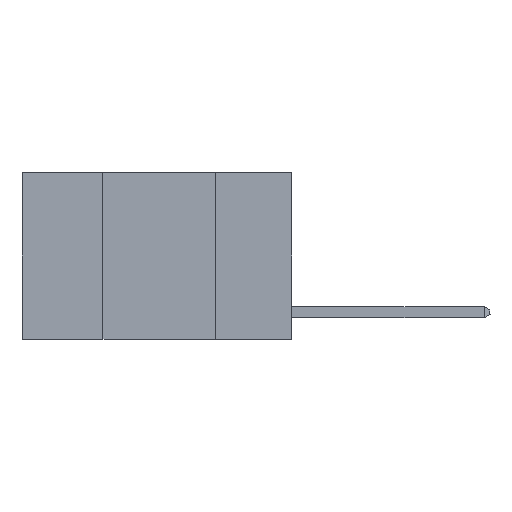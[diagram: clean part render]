
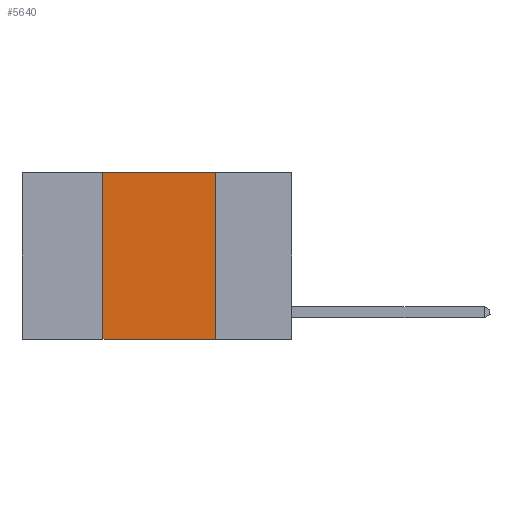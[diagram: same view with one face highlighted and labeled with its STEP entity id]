
A CAD part, left-side view. The second image highlights one B-rep face of the part: STEP entity #5640.
In plain terms, the highlighted planar face has unit normal (-1, 0, 0).
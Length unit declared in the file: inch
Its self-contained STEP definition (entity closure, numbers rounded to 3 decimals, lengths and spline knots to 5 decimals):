
#360 = EDGE_CURVE ( 'NONE', #12154, #3859, #1689, .T. ) ;
#563 = PLANE ( 'NONE',  #15640 ) ;
#622 = CARTESIAN_POINT ( 'NONE',  ( 0., 0.6, 0. ) ) ;
#1076 = DIRECTION ( 'NONE',  ( 0., 0., -1. ) ) ;
#1689 = LINE ( 'NONE', #13820, #8834 ) ;
#1871 = ORIENTED_EDGE ( 'NONE', *, *, #8017, .F. ) ;
#1886 = FACE_OUTER_BOUND ( 'NONE', #17137, .T. ) ;
#2322 = ORIENTED_EDGE ( 'NONE', *, *, #3202, .F. ) ;
#3202 = EDGE_CURVE ( 'NONE', #12154, #18218, #9195, .T. ) ;
#3463 = DIRECTION ( 'NONE',  ( 0., 0., -1. ) ) ;
#3859 = VERTEX_POINT ( 'NONE', #6863 ) ;
#5022 = CARTESIAN_POINT ( 'NONE',  ( 0., 0.42, 0. ) ) ;
#5640 = ADVANCED_FACE ( 'NONE', ( #1886 ), #563, .F. ) ;
#6737 = LINE ( 'NONE', #11041, #16740 ) ;
#6863 = CARTESIAN_POINT ( 'NONE',  ( 0., 0.17, -0.37 ) ) ;
#7523 = VERTEX_POINT ( 'NONE', #17915 ) ;
#8017 = EDGE_CURVE ( 'NONE', #7523, #3859, #6737, .T. ) ;
#8312 = LINE ( 'NONE', #13967, #15408 ) ;
#8834 = VECTOR ( 'NONE', #14888, 39.37008 ) ;
#9195 = LINE ( 'NONE', #5022, #16290 ) ;
#9756 = CARTESIAN_POINT ( 'NONE',  ( 0., 0.42, 0. ) ) ;
#11041 = CARTESIAN_POINT ( 'NONE',  ( 0., 0.17, 0. ) ) ;
#12005 = DIRECTION ( 'NONE',  ( 1., 0., 0. ) ) ;
#12154 = VERTEX_POINT ( 'NONE', #16333 ) ;
#12929 = EDGE_CURVE ( 'NONE', #18218, #7523, #8312, .T. ) ;
#13820 = CARTESIAN_POINT ( 'NONE',  ( 0., 0.6, -0.37 ) ) ;
#13887 = DIRECTION ( 'NONE',  ( 0., 0., 1. ) ) ;
#13967 = CARTESIAN_POINT ( 'NONE',  ( 0., 0.6, 0. ) ) ;
#14888 = DIRECTION ( 'NONE',  ( 0., -1., 0. ) ) ;
#15386 = DIRECTION ( 'NONE',  ( 0., -1., 0. ) ) ;
#15408 = VECTOR ( 'NONE', #15386, 39.37008 ) ;
#15640 = AXIS2_PLACEMENT_3D ( 'NONE', #622, #12005, #3463 ) ;
#16290 = VECTOR ( 'NONE', #13887, 39.37008 ) ;
#16333 = CARTESIAN_POINT ( 'NONE',  ( 0., 0.42, -0.37 ) ) ;
#16740 = VECTOR ( 'NONE', #1076, 39.37008 ) ;
#17029 = ORIENTED_EDGE ( 'NONE', *, *, #12929, .F. ) ;
#17137 = EDGE_LOOP ( 'NONE', ( #1871, #17029, #2322, #17459 ) ) ;
#17459 = ORIENTED_EDGE ( 'NONE', *, *, #360, .T. ) ;
#17915 = CARTESIAN_POINT ( 'NONE',  ( 0., 0.17, 0. ) ) ;
#18218 = VERTEX_POINT ( 'NONE', #9756 ) ;
